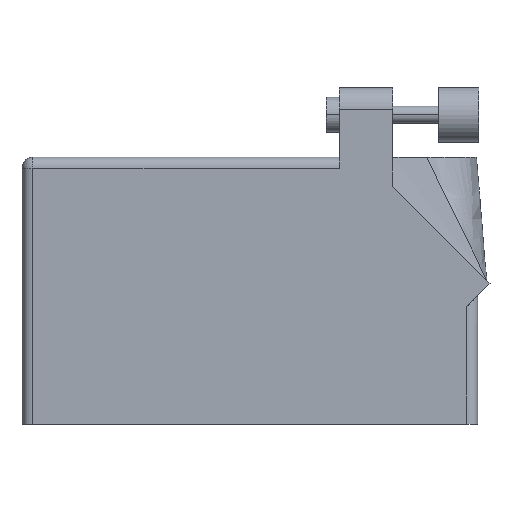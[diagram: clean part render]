
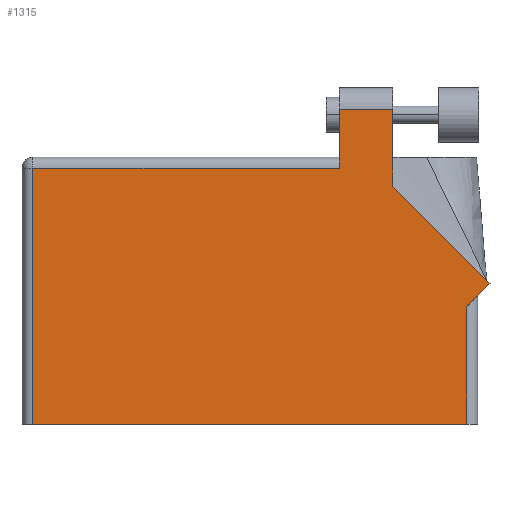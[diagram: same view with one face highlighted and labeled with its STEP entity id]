
A CAD part, top view. The second image highlights one B-rep face of the part: STEP entity #1315.
In plain terms, the highlighted planar face has unit normal (0, 0, 1).
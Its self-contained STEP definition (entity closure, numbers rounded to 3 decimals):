
#6 = DIRECTION ( 'NONE',  ( -1., 0., 0. ) ) ;
#33 = VERTEX_POINT ( 'NONE', #1217 ) ;
#70 = PLANE ( 'NONE',  #1917 ) ;
#84 = DIRECTION ( 'NONE',  ( 0., 0., -1. ) ) ;
#115 = ORIENTED_EDGE ( 'NONE', *, *, #2290, .T. ) ;
#117 = LINE ( 'NONE', #2020, #2411 ) ;
#193 = CARTESIAN_POINT ( 'NONE',  ( 54., 34.656, 0. ) ) ;
#240 = LINE ( 'NONE', #1383, #1492 ) ;
#282 = EDGE_LOOP ( 'NONE', ( #377, #2268, #1191, #435, #553, #1201, #1507, #1088, #115 ) ) ;
#330 = CARTESIAN_POINT ( 'NONE',  ( 54., 45.847, 0. ) ) ;
#352 = VERTEX_POINT ( 'NONE', #2259 ) ;
#377 = ORIENTED_EDGE ( 'NONE', *, *, #2502, .T. ) ;
#398 = DIRECTION ( 'NONE',  ( 0., -1., 0. ) ) ;
#435 = ORIENTED_EDGE ( 'NONE', *, *, #473, .T. ) ;
#473 = EDGE_CURVE ( 'NONE', #2356, #519, #1421, .T. ) ;
#519 = VERTEX_POINT ( 'NONE', #896 ) ;
#547 = VERTEX_POINT ( 'NONE', #2199 ) ;
#548 = VECTOR ( 'NONE', #1467, 1000. ) ;
#553 = ORIENTED_EDGE ( 'NONE', *, *, #906, .T. ) ;
#626 = EDGE_CURVE ( 'NONE', #352, #1808, #2423, .T. ) ;
#629 = DIRECTION ( 'NONE',  ( 1., 0., 0. ) ) ;
#639 = CARTESIAN_POINT ( 'NONE',  ( 54., 34.656, 0. ) ) ;
#642 = LINE ( 'NONE', #654, #796 ) ;
#654 = CARTESIAN_POINT ( 'NONE',  ( 0., 0., 0. ) ) ;
#703 = CARTESIAN_POINT ( 'NONE',  ( 66.345, 18.72, 0. ) ) ;
#729 = VECTOR ( 'NONE', #6, 1000. ) ;
#796 = VECTOR ( 'NONE', #629, 1000. ) ;
#834 = EDGE_CURVE ( 'NONE', #1197, #352, #1567, .T. ) ;
#878 = DIRECTION ( 'NONE',  ( -1., 0., 0. ) ) ;
#896 = CARTESIAN_POINT ( 'NONE',  ( 1.575, 37.287, 0. ) ) ;
#906 = EDGE_CURVE ( 'NONE', #519, #547, #240, .T. ) ;
#930 = DIRECTION ( 'NONE',  ( -1., 0., 0. ) ) ;
#948 = DIRECTION ( 'NONE',  ( 0., 1., 0. ) ) ;
#1030 = DIRECTION ( 'NONE',  ( 0., -1., 0. ) ) ;
#1088 = ORIENTED_EDGE ( 'NONE', *, *, #626, .T. ) ;
#1137 = LINE ( 'NONE', #193, #1560 ) ;
#1147 = VERTEX_POINT ( 'NONE', #330 ) ;
#1191 = ORIENTED_EDGE ( 'NONE', *, *, #2263, .T. ) ;
#1197 = VERTEX_POINT ( 'NONE', #1585 ) ;
#1201 = ORIENTED_EDGE ( 'NONE', *, *, #1738, .T. ) ;
#1217 = CARTESIAN_POINT ( 'NONE',  ( 46.203, 45.847, 0. ) ) ;
#1315 = ADVANCED_FACE ( 'NONE', ( #2016 ), #70, .F. ) ;
#1379 = CARTESIAN_POINT ( 'NONE',  ( 0., 37.287, 0. ) ) ;
#1383 = CARTESIAN_POINT ( 'NONE',  ( 1.575, 0., 0. ) ) ;
#1421 = LINE ( 'NONE', #1379, #729 ) ;
#1467 = DIRECTION ( 'NONE',  ( -0.707, 0.707, 0. ) ) ;
#1492 = VECTOR ( 'NONE', #398, 1000. ) ;
#1507 = ORIENTED_EDGE ( 'NONE', *, *, #834, .T. ) ;
#1560 = VECTOR ( 'NONE', #948, 1000. ) ;
#1567 = LINE ( 'NONE', #2355, #2180 ) ;
#1585 = CARTESIAN_POINT ( 'NONE',  ( 64.77, 0., 0. ) ) ;
#1738 = EDGE_CURVE ( 'NONE', #547, #1197, #642, .T. ) ;
#1743 = LINE ( 'NONE', #2319, #2408 ) ;
#1799 = CARTESIAN_POINT ( 'NONE',  ( 68.141, 20.516, 0. ) ) ;
#1808 = VERTEX_POINT ( 'NONE', #1799 ) ;
#1816 = CARTESIAN_POINT ( 'NONE',  ( 68.141, 20.516, 0. ) ) ;
#1825 = LINE ( 'NONE', #1816, #548 ) ;
#1856 = DIRECTION ( 'NONE',  ( 0.707, 0.707, 0. ) ) ;
#1917 = AXIS2_PLACEMENT_3D ( 'NONE', #1991, #84, #878 ) ;
#1991 = CARTESIAN_POINT ( 'NONE',  ( 0., 38.862, 0. ) ) ;
#2016 = FACE_OUTER_BOUND ( 'NONE', #282, .T. ) ;
#2020 = CARTESIAN_POINT ( 'NONE',  ( 46.203, 38.862, 0. ) ) ;
#2084 = EDGE_CURVE ( 'NONE', #1147, #33, #1743, .T. ) ;
#2164 = VERTEX_POINT ( 'NONE', #639 ) ;
#2180 = VECTOR ( 'NONE', #2317, 1000. ) ;
#2199 = CARTESIAN_POINT ( 'NONE',  ( 1.575, 0., 0. ) ) ;
#2211 = CARTESIAN_POINT ( 'NONE',  ( 46.203, 37.287, 0. ) ) ;
#2259 = CARTESIAN_POINT ( 'NONE',  ( 64.77, 17.145, 0. ) ) ;
#2263 = EDGE_CURVE ( 'NONE', #33, #2356, #117, .T. ) ;
#2268 = ORIENTED_EDGE ( 'NONE', *, *, #2084, .T. ) ;
#2290 = EDGE_CURVE ( 'NONE', #1808, #2164, #1825, .T. ) ;
#2317 = DIRECTION ( 'NONE',  ( 0., 1., 0. ) ) ;
#2319 = CARTESIAN_POINT ( 'NONE',  ( 46.203, 45.847, 0. ) ) ;
#2355 = CARTESIAN_POINT ( 'NONE',  ( 64.77, 18.72, 0. ) ) ;
#2356 = VERTEX_POINT ( 'NONE', #2211 ) ;
#2408 = VECTOR ( 'NONE', #930, 1000. ) ;
#2411 = VECTOR ( 'NONE', #1030, 1000. ) ;
#2423 = LINE ( 'NONE', #703, #2425 ) ;
#2425 = VECTOR ( 'NONE', #1856, 1000. ) ;
#2502 = EDGE_CURVE ( 'NONE', #2164, #1147, #1137, .T. ) ;
